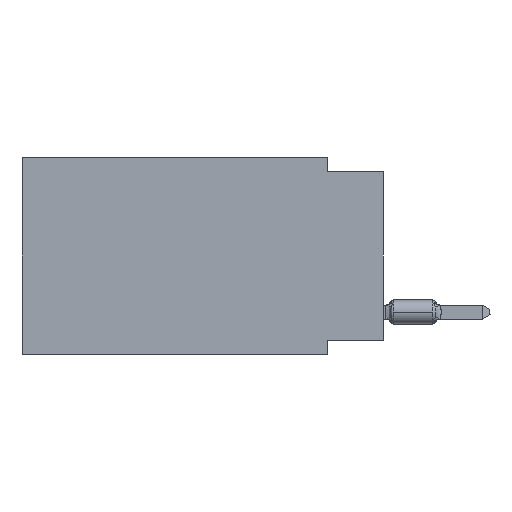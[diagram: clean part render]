
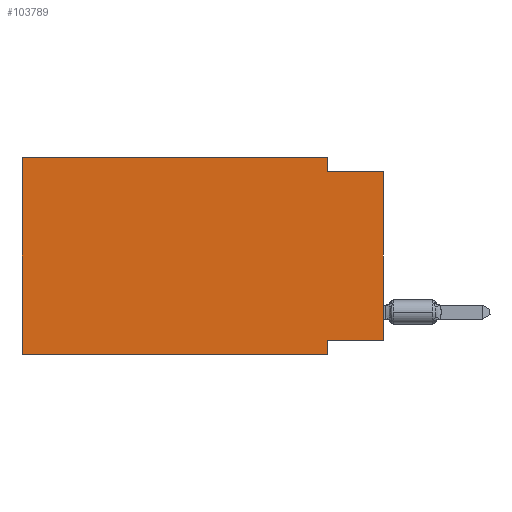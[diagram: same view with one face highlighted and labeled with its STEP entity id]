
A CAD part, left-side view. The second image highlights one B-rep face of the part: STEP entity #103789.
In plain terms, the highlighted planar face has unit normal (-1, 0, 0).
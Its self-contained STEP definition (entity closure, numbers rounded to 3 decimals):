
#702 = LINE ( 'NONE', #19583, #12520 ) ;
#1804 = CARTESIAN_POINT ( 'NONE',  ( 0., 16.383, 0. ) ) ;
#2833 = DIRECTION ( 'NONE',  ( 0., 0., -1. ) ) ;
#2973 = CARTESIAN_POINT ( 'NONE',  ( 0., 2.54, 0. ) ) ;
#6198 = EDGE_CURVE ( 'NONE', #79592, #36528, #99586, .T. ) ;
#9833 = DIRECTION ( 'NONE',  ( 0., -1., 0. ) ) ;
#10324 = CARTESIAN_POINT ( 'NONE',  ( 0., 2.54, -8.255 ) ) ;
#12101 = LINE ( 'NONE', #1804, #96706 ) ;
#12520 = VECTOR ( 'NONE', #36761, 1000. ) ;
#12660 = DIRECTION ( 'NONE',  ( 0., -1., 0. ) ) ;
#13736 = VECTOR ( 'NONE', #2833, 1000. ) ;
#14336 = EDGE_CURVE ( 'NONE', #83691, #104314, #12101, .T. ) ;
#16755 = CARTESIAN_POINT ( 'NONE',  ( 0., 0., -0.635 ) ) ;
#17232 = VECTOR ( 'NONE', #81786, 1000. ) ;
#19583 = CARTESIAN_POINT ( 'NONE',  ( 0., 0., 0. ) ) ;
#20156 = VECTOR ( 'NONE', #75738, 1000. ) ;
#20537 = CARTESIAN_POINT ( 'NONE',  ( 0., 16.383, -8.89 ) ) ;
#24175 = VECTOR ( 'NONE', #113287, 1000. ) ;
#24206 = EDGE_CURVE ( 'NONE', #95021, #36528, #98969, .T. ) ;
#24951 = EDGE_CURVE ( 'NONE', #66853, #36606, #96330, .T. ) ;
#34573 = EDGE_CURVE ( 'NONE', #95021, #83691, #66447, .T. ) ;
#34670 = DIRECTION ( 'NONE',  ( 0., 0., -1. ) ) ;
#36528 = VERTEX_POINT ( 'NONE', #58119 ) ;
#36606 = VERTEX_POINT ( 'NONE', #100488 ) ;
#36761 = DIRECTION ( 'NONE',  ( 0., 0., 1. ) ) ;
#49267 = DIRECTION ( 'NONE',  ( 0., 0., 1. ) ) ;
#51276 = CARTESIAN_POINT ( 'NONE',  ( 0., 16.383, 0. ) ) ;
#52845 = EDGE_LOOP ( 'NONE', ( #80769, #83648, #84881, #101135, #81761, #81172, #60752, #107052 ) ) ;
#57879 = CARTESIAN_POINT ( 'NONE',  ( 0., 16.383, 0. ) ) ;
#58119 = CARTESIAN_POINT ( 'NONE',  ( 0., 2.54, -8.89 ) ) ;
#60740 = CARTESIAN_POINT ( 'NONE',  ( 0., 16.383, -8.89 ) ) ;
#60752 = ORIENTED_EDGE ( 'NONE', *, *, #6198, .F. ) ;
#62522 = EDGE_CURVE ( 'NONE', #69010, #79592, #102652, .T. ) ;
#62928 = VECTOR ( 'NONE', #49267, 1000. ) ;
#64911 = LINE ( 'NONE', #78320, #24175 ) ;
#66447 = LINE ( 'NONE', #57879, #62928 ) ;
#66853 = VERTEX_POINT ( 'NONE', #109309 ) ;
#69010 = VERTEX_POINT ( 'NONE', #96146 ) ;
#72687 = CARTESIAN_POINT ( 'NONE',  ( 0., 2.54, -8.89 ) ) ;
#75738 = DIRECTION ( 'NONE',  ( 0., 1., 0. ) ) ;
#78320 = CARTESIAN_POINT ( 'NONE',  ( 0., 2.54, 0. ) ) ;
#79592 = VERTEX_POINT ( 'NONE', #10324 ) ;
#79757 = VECTOR ( 'NONE', #9833, 1000. ) ;
#80769 = ORIENTED_EDGE ( 'NONE', *, *, #103083, .T. ) ;
#81172 = ORIENTED_EDGE ( 'NONE', *, *, #24206, .T. ) ;
#81761 = ORIENTED_EDGE ( 'NONE', *, *, #34573, .F. ) ;
#81786 = DIRECTION ( 'NONE',  ( 0., -1., 0. ) ) ;
#83648 = ORIENTED_EDGE ( 'NONE', *, *, #24951, .F. ) ;
#83691 = VERTEX_POINT ( 'NONE', #106918 ) ;
#84881 = ORIENTED_EDGE ( 'NONE', *, *, #94214, .F. ) ;
#87559 = AXIS2_PLACEMENT_3D ( 'NONE', #51276, #93684, #34670 ) ;
#93497 = CARTESIAN_POINT ( 'NONE',  ( 0., 0., -8.255 ) ) ;
#93684 = DIRECTION ( 'NONE',  ( 1., 0., 0. ) ) ;
#94214 = EDGE_CURVE ( 'NONE', #104314, #66853, #64911, .T. ) ;
#95021 = VERTEX_POINT ( 'NONE', #60740 ) ;
#95938 = FACE_OUTER_BOUND ( 'NONE', #52845, .T. ) ;
#96146 = CARTESIAN_POINT ( 'NONE',  ( 0., 0., -8.255 ) ) ;
#96330 = LINE ( 'NONE', #16755, #79757 ) ;
#96706 = VECTOR ( 'NONE', #12660, 1000. ) ;
#98969 = LINE ( 'NONE', #20537, #17232 ) ;
#99586 = LINE ( 'NONE', #72687, #13736 ) ;
#100488 = CARTESIAN_POINT ( 'NONE',  ( 0., 0., -0.635 ) ) ;
#101135 = ORIENTED_EDGE ( 'NONE', *, *, #14336, .F. ) ;
#102652 = LINE ( 'NONE', #93497, #20156 ) ;
#103083 = EDGE_CURVE ( 'NONE', #69010, #36606, #702, .T. ) ;
#103393 = PLANE ( 'NONE',  #87559 ) ;
#103789 = ADVANCED_FACE ( 'NONE', ( #95938 ), #103393, .F. ) ;
#104314 = VERTEX_POINT ( 'NONE', #2973 ) ;
#106918 = CARTESIAN_POINT ( 'NONE',  ( 0., 16.383, 0. ) ) ;
#107052 = ORIENTED_EDGE ( 'NONE', *, *, #62522, .F. ) ;
#109309 = CARTESIAN_POINT ( 'NONE',  ( 0., 2.54, -0.635 ) ) ;
#113287 = DIRECTION ( 'NONE',  ( 0., 0., -1. ) ) ;
